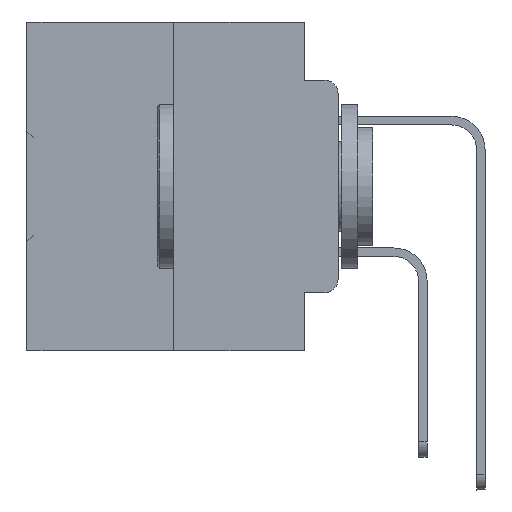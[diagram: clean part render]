
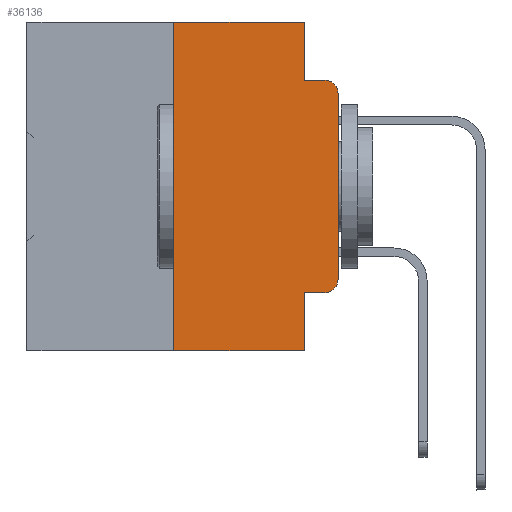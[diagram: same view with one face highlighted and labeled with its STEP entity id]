
A CAD part, left-side view. The second image highlights one B-rep face of the part: STEP entity #36136.
In plain terms, the highlighted planar face has unit normal (-1, 0, 0).
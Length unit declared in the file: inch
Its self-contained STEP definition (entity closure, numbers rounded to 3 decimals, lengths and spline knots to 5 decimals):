
#720 = CARTESIAN_POINT ( 'NONE',  ( 0., 0.25, 0. ) ) ;
#1127 = VECTOR ( 'NONE', #24312, 39.37008 ) ;
#1216 = CIRCLE ( 'NONE', #14482, 0.02 ) ;
#1560 = CIRCLE ( 'NONE', #17107, 0.02 ) ;
#1601 = ORIENTED_EDGE ( 'NONE', *, *, #26006, .F. ) ;
#2316 = VERTEX_POINT ( 'NONE', #36148 ) ;
#2512 = VERTEX_POINT ( 'NONE', #35249 ) ;
#3077 = CARTESIAN_POINT ( 'NONE',  ( 0., 0.051, 0. ) ) ;
#3966 = PLANE ( 'NONE',  #28030 ) ;
#4031 = CARTESIAN_POINT ( 'NONE',  ( 0., 0.051, -0.0885 ) ) ;
#4550 = VERTEX_POINT ( 'NONE', #14333 ) ;
#5687 = CARTESIAN_POINT ( 'NONE',  ( 0., 0.25, 0. ) ) ;
#6162 = VECTOR ( 'NONE', #34834, 39.37008 ) ;
#8156 = VECTOR ( 'NONE', #25394, 39.37008 ) ;
#8263 = VECTOR ( 'NONE', #9181, 39.37008 ) ;
#8457 = ORIENTED_EDGE ( 'NONE', *, *, #31176, .T. ) ;
#9181 = DIRECTION ( 'NONE',  ( 0., 0., -1. ) ) ;
#9236 = LINE ( 'NONE', #30332, #8263 ) ;
#9490 = CARTESIAN_POINT ( 'NONE',  ( 0., 0.02, -0.4115 ) ) ;
#9520 = CARTESIAN_POINT ( 'NONE',  ( 0., 0.02, -0.1085 ) ) ;
#9602 = VERTEX_POINT ( 'NONE', #11722 ) ;
#10196 = DIRECTION ( 'NONE',  ( 0., 0., -1. ) ) ;
#10431 = ORIENTED_EDGE ( 'NONE', *, *, #33951, .T. ) ;
#10959 = EDGE_CURVE ( 'NONE', #24277, #22862, #32450, .T. ) ;
#11369 = ORIENTED_EDGE ( 'NONE', *, *, #15039, .F. ) ;
#11722 = CARTESIAN_POINT ( 'NONE',  ( 0., 0., -0.3915 ) ) ;
#13012 = EDGE_CURVE ( 'NONE', #4550, #32792, #26960, .T. ) ;
#13135 = DIRECTION ( 'NONE',  ( 0., 0., -1. ) ) ;
#14324 = CARTESIAN_POINT ( 'NONE',  ( 0., 0.02, -0.3915 ) ) ;
#14333 = CARTESIAN_POINT ( 'NONE',  ( 0., 0.25, -0.5 ) ) ;
#14482 = AXIS2_PLACEMENT_3D ( 'NONE', #9520, #31168, #13135 ) ;
#14575 = CARTESIAN_POINT ( 'NONE',  ( 0., 0.051, -0.4115 ) ) ;
#15039 = EDGE_CURVE ( 'NONE', #34037, #35326, #9236, .T. ) ;
#15446 = VECTOR ( 'NONE', #39279, 39.37008 ) ;
#15669 = ORIENTED_EDGE ( 'NONE', *, *, #35954, .T. ) ;
#17075 = EDGE_CURVE ( 'NONE', #35326, #2512, #39283, .T. ) ;
#17107 = AXIS2_PLACEMENT_3D ( 'NONE', #14324, #35367, #17394 ) ;
#17394 = DIRECTION ( 'NONE',  ( 0., 0., -1. ) ) ;
#17599 = LINE ( 'NONE', #33177, #1127 ) ;
#18057 = ORIENTED_EDGE ( 'NONE', *, *, #13012, .F. ) ;
#18419 = DIRECTION ( 'NONE',  ( 0., 0., -1. ) ) ;
#19501 = LINE ( 'NONE', #25915, #26555 ) ;
#19950 = ORIENTED_EDGE ( 'NONE', *, *, #20925, .T. ) ;
#20925 = EDGE_CURVE ( 'NONE', #4550, #22862, #17599, .T. ) ;
#21560 = CARTESIAN_POINT ( 'NONE',  ( 0., 0.051, -0.0885 ) ) ;
#22415 = LINE ( 'NONE', #31832, #6162 ) ;
#22862 = VERTEX_POINT ( 'NONE', #33297 ) ;
#23240 = ORIENTED_EDGE ( 'NONE', *, *, #33208, .T. ) ;
#23638 = CARTESIAN_POINT ( 'NONE',  ( 0., 0.051, 0. ) ) ;
#24277 = VERTEX_POINT ( 'NONE', #14575 ) ;
#24312 = DIRECTION ( 'NONE',  ( 0., -1., 0. ) ) ;
#24538 = VECTOR ( 'NONE', #18419, 39.37008 ) ;
#24666 = ORIENTED_EDGE ( 'NONE', *, *, #17075, .F. ) ;
#25329 = CARTESIAN_POINT ( 'NONE',  ( 0., 0.473, 0. ) ) ;
#25358 = DIRECTION ( 'NONE',  ( 0., 0., 1. ) ) ;
#25394 = DIRECTION ( 'NONE',  ( 0., -1., 0. ) ) ;
#25868 = FACE_OUTER_BOUND ( 'NONE', #29196, .T. ) ;
#25915 = CARTESIAN_POINT ( 'NONE',  ( 0., 0., 0. ) ) ;
#26006 = EDGE_CURVE ( 'NONE', #32792, #34037, #22415, .T. ) ;
#26555 = VECTOR ( 'NONE', #28925, 39.37008 ) ;
#26960 = LINE ( 'NONE', #720, #32087 ) ;
#28030 = AXIS2_PLACEMENT_3D ( 'NONE', #25329, #28329, #10196 ) ;
#28329 = DIRECTION ( 'NONE',  ( 1., 0., 0. ) ) ;
#28925 = DIRECTION ( 'NONE',  ( 0., 0., 1. ) ) ;
#29196 = EDGE_LOOP ( 'NONE', ( #23240, #8457, #24666, #11369, #1601, #18057, #19950, #36839, #15669, #10431 ) ) ;
#30332 = CARTESIAN_POINT ( 'NONE',  ( 0., 0.051, 0. ) ) ;
#30409 = CARTESIAN_POINT ( 'NONE',  ( 0., 0.051, -0.4115 ) ) ;
#31168 = DIRECTION ( 'NONE',  ( -1., 0., 0. ) ) ;
#31176 = EDGE_CURVE ( 'NONE', #2316, #2512, #1216, .T. ) ;
#31832 = CARTESIAN_POINT ( 'NONE',  ( 0., 0.473, 0. ) ) ;
#32087 = VECTOR ( 'NONE', #25358, 39.37008 ) ;
#32399 = LINE ( 'NONE', #30409, #15446 ) ;
#32450 = LINE ( 'NONE', #3077, #24538 ) ;
#32792 = VERTEX_POINT ( 'NONE', #5687 ) ;
#33177 = CARTESIAN_POINT ( 'NONE',  ( 0., 0.473, -0.5 ) ) ;
#33208 = EDGE_CURVE ( 'NONE', #9602, #2316, #19501, .T. ) ;
#33297 = CARTESIAN_POINT ( 'NONE',  ( 0., 0.051, -0.5 ) ) ;
#33951 = EDGE_CURVE ( 'NONE', #34700, #9602, #1560, .T. ) ;
#34037 = VERTEX_POINT ( 'NONE', #23638 ) ;
#34700 = VERTEX_POINT ( 'NONE', #9490 ) ;
#34834 = DIRECTION ( 'NONE',  ( 0., -1., 0. ) ) ;
#35249 = CARTESIAN_POINT ( 'NONE',  ( 0., 0.02, -0.0885 ) ) ;
#35326 = VERTEX_POINT ( 'NONE', #21560 ) ;
#35367 = DIRECTION ( 'NONE',  ( -1., 0., 0. ) ) ;
#35954 = EDGE_CURVE ( 'NONE', #24277, #34700, #32399, .T. ) ;
#36136 = ADVANCED_FACE ( 'NONE', ( #25868 ), #3966, .F. ) ;
#36148 = CARTESIAN_POINT ( 'NONE',  ( 0., 0., -0.1085 ) ) ;
#36839 = ORIENTED_EDGE ( 'NONE', *, *, #10959, .F. ) ;
#39279 = DIRECTION ( 'NONE',  ( 0., -1., 0. ) ) ;
#39283 = LINE ( 'NONE', #4031, #8156 ) ;
